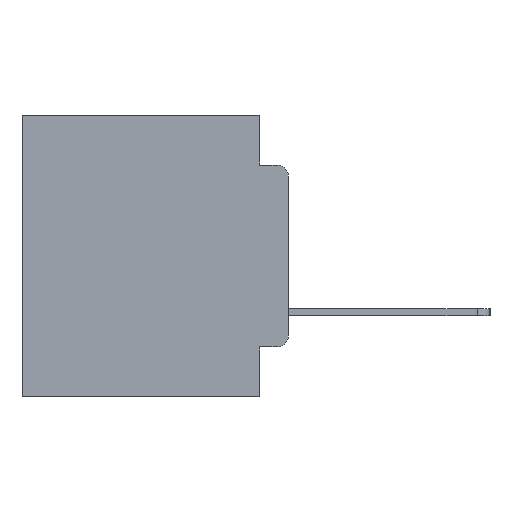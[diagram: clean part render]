
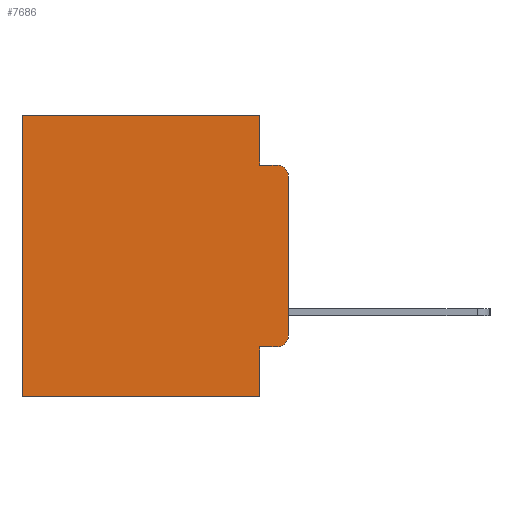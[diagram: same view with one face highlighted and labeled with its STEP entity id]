
A CAD part, left-side view. The second image highlights one B-rep face of the part: STEP entity #7686.
In plain terms, the highlighted planar face has unit normal (-1, 0, 0).
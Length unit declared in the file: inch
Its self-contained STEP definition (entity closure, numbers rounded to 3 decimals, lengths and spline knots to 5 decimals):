
#374 = EDGE_CURVE ( 'NONE', #19818, #2035, #9308, .T. ) ;
#1035 = DIRECTION ( 'NONE',  ( 0., 0., -1. ) ) ;
#1221 = VERTEX_POINT ( 'NONE', #16633 ) ;
#1318 = VECTOR ( 'NONE', #13589, 39.37008 ) ;
#1697 = AXIS2_PLACEMENT_3D ( 'NONE', #3186, #17403, #5242 ) ;
#1820 = VERTEX_POINT ( 'NONE', #23166 ) ;
#1821 = CARTESIAN_POINT ( 'NONE',  ( 0.298, 0., -0.5 ) ) ;
#2035 = VERTEX_POINT ( 'NONE', #5546 ) ;
#2037 = PLANE ( 'NONE',  #12512 ) ;
#2078 = DIRECTION ( 'NONE',  ( 0., 0., -1. ) ) ;
#2272 = LINE ( 'NONE', #1821, #21839 ) ;
#2429 = LINE ( 'NONE', #16990, #23215 ) ;
#3068 = EDGE_CURVE ( 'NONE', #19818, #15734, #12236, .T. ) ;
#3186 = CARTESIAN_POINT ( 'NONE',  ( 0.298, 0.02, -0.3915 ) ) ;
#3294 = CARTESIAN_POINT ( 'NONE',  ( 0.298, 0., 0. ) ) ;
#3416 = CARTESIAN_POINT ( 'NONE',  ( 0.298, 0.051, -0.0885 ) ) ;
#3743 = VECTOR ( 'NONE', #15460, 39.37008 ) ;
#4002 = CARTESIAN_POINT ( 'NONE',  ( 0.298, 0., -0.1085 ) ) ;
#4601 = AXIS2_PLACEMENT_3D ( 'NONE', #15303, #24400, #25055 ) ;
#5129 = EDGE_CURVE ( 'NONE', #6109, #13298, #5329, .T. ) ;
#5175 = CIRCLE ( 'NONE', #1697, 0.02 ) ;
#5242 = DIRECTION ( 'NONE',  ( 0., 0., -1. ) ) ;
#5329 = LINE ( 'NONE', #5710, #10217 ) ;
#5546 = CARTESIAN_POINT ( 'NONE',  ( 0.298, 0.02, -0.0885 ) ) ;
#5579 = VERTEX_POINT ( 'NONE', #25078 ) ;
#5710 = CARTESIAN_POINT ( 'NONE',  ( 0.298, 0., 0. ) ) ;
#6109 = VERTEX_POINT ( 'NONE', #9130 ) ;
#6130 = DIRECTION ( 'NONE',  ( 0., 0., -1. ) ) ;
#6581 = ORIENTED_EDGE ( 'NONE', *, *, #23776, .F. ) ;
#7545 = VECTOR ( 'NONE', #23562, 39.37008 ) ;
#7686 = ADVANCED_FACE ( 'NONE', ( #16350 ), #2037, .F. ) ;
#8680 = CARTESIAN_POINT ( 'NONE',  ( 0.298, 0.051, -0.5 ) ) ;
#8716 = EDGE_LOOP ( 'NONE', ( #16103, #16736, #22010, #6581, #12704, #17961, #24408, #14565, #15196, #10487 ) ) ;
#9117 = EDGE_CURVE ( 'NONE', #14062, #15734, #5175, .T. ) ;
#9130 = CARTESIAN_POINT ( 'NONE',  ( 0.298, 0.051, 0. ) ) ;
#9216 = LINE ( 'NONE', #25036, #19199 ) ;
#9308 = CIRCLE ( 'NONE', #4601, 0.02 ) ;
#10217 = VECTOR ( 'NONE', #11966, 39.37008 ) ;
#10487 = ORIENTED_EDGE ( 'NONE', *, *, #9117, .T. ) ;
#11073 = DIRECTION ( 'NONE',  ( 0., 0., -1. ) ) ;
#11662 = LINE ( 'NONE', #20192, #20938 ) ;
#11966 = DIRECTION ( 'NONE',  ( 0., 1., 0. ) ) ;
#12236 = LINE ( 'NONE', #3294, #1318 ) ;
#12512 = AXIS2_PLACEMENT_3D ( 'NONE', #16264, #18229, #6130 ) ;
#12704 = ORIENTED_EDGE ( 'NONE', *, *, #5129, .T. ) ;
#13298 = VERTEX_POINT ( 'NONE', #19519 ) ;
#13589 = DIRECTION ( 'NONE',  ( 0., 0., -1. ) ) ;
#14062 = VERTEX_POINT ( 'NONE', #25202 ) ;
#14565 = ORIENTED_EDGE ( 'NONE', *, *, #17196, .F. ) ;
#15196 = ORIENTED_EDGE ( 'NONE', *, *, #15863, .T. ) ;
#15303 = CARTESIAN_POINT ( 'NONE',  ( 0.298, 0.02, -0.1085 ) ) ;
#15460 = DIRECTION ( 'NONE',  ( 0., -1., 0. ) ) ;
#15734 = VERTEX_POINT ( 'NONE', #24721 ) ;
#15863 = EDGE_CURVE ( 'NONE', #5579, #14062, #19881, .T. ) ;
#16103 = ORIENTED_EDGE ( 'NONE', *, *, #3068, .F. ) ;
#16264 = CARTESIAN_POINT ( 'NONE',  ( 0.298, 0., 0. ) ) ;
#16350 = FACE_OUTER_BOUND ( 'NONE', #8716, .T. ) ;
#16633 = CARTESIAN_POINT ( 'NONE',  ( 0.298, 0.051, -0.0885 ) ) ;
#16736 = ORIENTED_EDGE ( 'NONE', *, *, #374, .T. ) ;
#16990 = CARTESIAN_POINT ( 'NONE',  ( 0.298, 0.051, 0. ) ) ;
#17196 = EDGE_CURVE ( 'NONE', #5579, #20602, #2429, .T. ) ;
#17403 = DIRECTION ( 'NONE',  ( -1., 0., 0. ) ) ;
#17961 = ORIENTED_EDGE ( 'NONE', *, *, #19827, .T. ) ;
#18023 = DIRECTION ( 'NONE',  ( 0., 1., 0. ) ) ;
#18229 = DIRECTION ( 'NONE',  ( 1., 0., 0. ) ) ;
#19199 = VECTOR ( 'NONE', #1035, 39.37008 ) ;
#19519 = CARTESIAN_POINT ( 'NONE',  ( 0.298, 0.473, 0. ) ) ;
#19818 = VERTEX_POINT ( 'NONE', #4002 ) ;
#19827 = EDGE_CURVE ( 'NONE', #13298, #1820, #11662, .T. ) ;
#19881 = LINE ( 'NONE', #23397, #3743 ) ;
#20192 = CARTESIAN_POINT ( 'NONE',  ( 0.298, 0.473, 0. ) ) ;
#20602 = VERTEX_POINT ( 'NONE', #8680 ) ;
#20938 = VECTOR ( 'NONE', #2078, 39.37008 ) ;
#21531 = EDGE_CURVE ( 'NONE', #20602, #1820, #2272, .T. ) ;
#21839 = VECTOR ( 'NONE', #18023, 39.37008 ) ;
#22010 = ORIENTED_EDGE ( 'NONE', *, *, #25049, .F. ) ;
#23166 = CARTESIAN_POINT ( 'NONE',  ( 0.298, 0.473, -0.5 ) ) ;
#23215 = VECTOR ( 'NONE', #11073, 39.37008 ) ;
#23397 = CARTESIAN_POINT ( 'NONE',  ( 0.298, 0.051, -0.4115 ) ) ;
#23500 = LINE ( 'NONE', #3416, #7545 ) ;
#23562 = DIRECTION ( 'NONE',  ( 0., -1., 0. ) ) ;
#23776 = EDGE_CURVE ( 'NONE', #6109, #1221, #9216, .T. ) ;
#24400 = DIRECTION ( 'NONE',  ( -1., 0., 0. ) ) ;
#24408 = ORIENTED_EDGE ( 'NONE', *, *, #21531, .F. ) ;
#24721 = CARTESIAN_POINT ( 'NONE',  ( 0.298, 0., -0.3915 ) ) ;
#25036 = CARTESIAN_POINT ( 'NONE',  ( 0.298, 0.051, 0. ) ) ;
#25049 = EDGE_CURVE ( 'NONE', #1221, #2035, #23500, .T. ) ;
#25055 = DIRECTION ( 'NONE',  ( 0., 0., -1. ) ) ;
#25078 = CARTESIAN_POINT ( 'NONE',  ( 0.298, 0.051, -0.4115 ) ) ;
#25202 = CARTESIAN_POINT ( 'NONE',  ( 0.298, 0.02, -0.4115 ) ) ;
